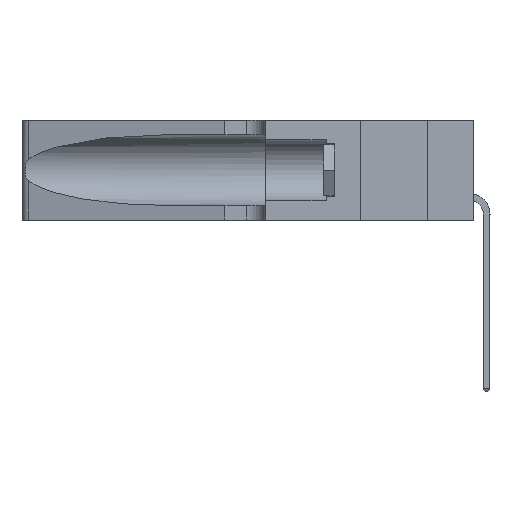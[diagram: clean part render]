
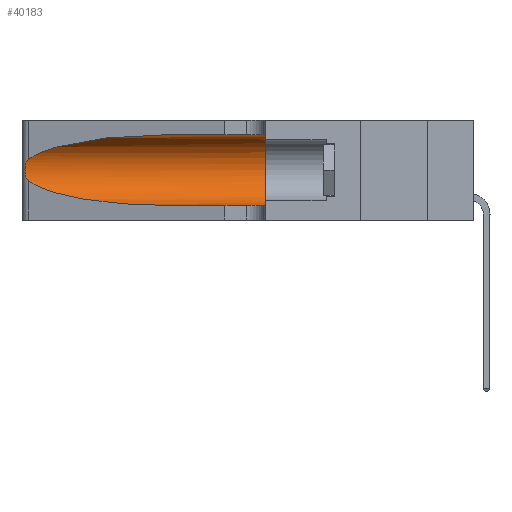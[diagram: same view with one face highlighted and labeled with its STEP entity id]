
A CAD part, left-side view. The second image highlights one B-rep face of the part: STEP entity #40183.
In plain terms, the highlighted cylindrical face has radius 3.308 mm (diameter 6.617 mm), a partial arc.
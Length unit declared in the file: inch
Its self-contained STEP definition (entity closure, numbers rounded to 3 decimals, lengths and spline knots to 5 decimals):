
#824 = LINE ( 'NONE', #29548, #28045 ) ;
#973 = CARTESIAN_POINT ( 'NONE',  ( 0.25487, 1.22718, 0.22369 ) ) ;
#1324 = VECTOR ( 'NONE', #36183, 39.37008 ) ;
#3163 = CARTESIAN_POINT ( 'NONE',  ( 0.25854, 1.2359, 0.20912 ) ) ;
#4702 = CARTESIAN_POINT ( 'NONE',  ( 0.1305, 0.35, 0.05475 ) ) ;
#4826 = ORIENTED_EDGE ( 'NONE', *, *, #31050, .T. ) ;
#7229 = CARTESIAN_POINT ( 'NONE',  ( 0.2373, 1.15595, 0.28018 ) ) ;
#8514 = LINE ( 'NONE', #33286, #1324 ) ;
#10471 = VERTEX_POINT ( 'NONE', #37526 ) ;
#10708 = CARTESIAN_POINT ( 'NONE',  ( 0.25487, 1.22718, 0.14631 ) ) ;
#12821 = DIRECTION ( 'NONE',  ( 0., 0., 1. ) ) ;
#12912 = CARTESIAN_POINT ( 'NONE',  ( 0.18966, 0.96281, 0.05475 ) ) ;
#12975 = CARTESIAN_POINT ( 'NONE',  ( 0.25487, 1.22718, 0.14631 ) ) ;
#13049 = CYLINDRICAL_SURFACE ( 'NONE', #17770, 0.13025 ) ;
#13206 = VERTEX_POINT ( 'NONE', #13548 ) ;
#13548 = CARTESIAN_POINT ( 'NONE',  ( 0.1305, 0.72297, 0.05475 ) ) ;
#15784 = ORIENTED_EDGE ( 'NONE', *, *, #37492, .F. ) ;
#16035 = CARTESIAN_POINT ( 'NONE',  ( 0.26075, 1.23896, 0.178 ) ) ;
#16224 = DIRECTION ( 'NONE',  ( 0., 0., -1. ) ) ;
#16693 = DIRECTION ( 'NONE',  ( 0., -1., 0. ) ) ;
#17770 = AXIS2_PLACEMENT_3D ( 'NONE', #26610, #35866, #16224 ) ;
#18976 = CARTESIAN_POINT ( 'NONE',  ( 0.1305, 0.72297, 0.05475 ) ) ;
#19411 = ORIENTED_EDGE ( 'NONE', *, *, #23525, .T. ) ;
#20201 = CARTESIAN_POINT ( 'NONE',  ( 0.18966, 0.96281, 0.31525 ) ) ;
#20498 = VERTEX_POINT ( 'NONE', #35727 ) ;
#20752 = VERTEX_POINT ( 'NONE', #4702 ) ;
#22020 = VERTEX_POINT ( 'NONE', #973 ) ;
#22325 = CARTESIAN_POINT ( 'NONE',  ( 0.25639, 1.23186, 0.15144 ) ) ;
#22878 = CARTESIAN_POINT ( 'NONE',  ( 0.1305, 0.35, 0.185 ) ) ;
#23478 = CARTESIAN_POINT ( 'NONE',  ( 0.1305, 0.72297, 0.31525 ) ) ;
#23525 = EDGE_CURVE ( 'NONE', #13206, #20752, #824, .T. ) ;
#25500 = EDGE_CURVE ( 'NONE', #20498, #22020, #26716, .T. ) ;
#25588 = CARTESIAN_POINT ( 'NONE',  ( 0.26017, 1.23833, 0.17102 ) ) ;
#25956 = CARTESIAN_POINT ( 'NONE',  ( 0.25487, 1.22718, 0.14631 ) ) ;
#26283 = DIRECTION ( 'NONE',  ( 0., 1., 0. ) ) ;
#26521 = ORIENTED_EDGE ( 'NONE', *, *, #36376, .T. ) ;
#26610 = CARTESIAN_POINT ( 'NONE',  ( 0.1305, 1.61858, 0.185 ) ) ;
#26619 = CARTESIAN_POINT ( 'NONE',  ( 0.25487, 1.22718, 0.22369 ) ) ;
#26694 = EDGE_CURVE ( 'NONE', #20498, #10471, #8514, .T. ) ;
#26716 =( BOUNDED_CURVE ( )  B_SPLINE_CURVE ( 3, ( #23478, #20201, #7229, #26619 ),
 .UNSPECIFIED., .F., .T. ) 
 B_SPLINE_CURVE_WITH_KNOTS ( ( 4, 4 ),
 ( 1.5708, 2.84003 ),
 .UNSPECIFIED. ) 
 CURVE ( )  GEOMETRIC_REPRESENTATION_ITEM ( )  RATIONAL_B_SPLINE_CURVE ( ( 1., 0.87, 0.87, 1. ) ) 
 REPRESENTATION_ITEM ( '' )  );
#27386 = FACE_OUTER_BOUND ( 'NONE', #37531, .T. ) ;
#27489 =( BOUNDED_CURVE ( )  B_SPLINE_CURVE ( 3, ( #25956, #42255, #12912, #18976 ),
 .UNSPECIFIED., .F., .T. ) 
 B_SPLINE_CURVE_WITH_KNOTS ( ( 4, 4 ),
 ( 3.44316, 4.71239 ),
 .UNSPECIFIED. ) 
 CURVE ( )  GEOMETRIC_REPRESENTATION_ITEM ( )  RATIONAL_B_SPLINE_CURVE ( ( 1., 0.87, 0.87, 1. ) ) 
 REPRESENTATION_ITEM ( '' )  );
#28045 = VECTOR ( 'NONE', #16693, 39.37008 ) ;
#28880 = CARTESIAN_POINT ( 'NONE',  ( 0.25555, 1.22994, 0.2215 ) ) ;
#29548 = CARTESIAN_POINT ( 'NONE',  ( 0.1305, 1.61858, 0.05475 ) ) ;
#30541 = ORIENTED_EDGE ( 'NONE', *, *, #26694, .F. ) ;
#31050 = EDGE_CURVE ( 'NONE', #22020, #38394, #36469, .T. ) ;
#32314 = ORIENTED_EDGE ( 'NONE', *, *, #25500, .T. ) ;
#32475 = CARTESIAN_POINT ( 'NONE',  ( 0.25789, 1.23486, 0.15765 ) ) ;
#32757 = CARTESIAN_POINT ( 'NONE',  ( 0.26075, 1.23896, 0.19203 ) ) ;
#33286 = CARTESIAN_POINT ( 'NONE',  ( 0.1305, 1.61858, 0.31525 ) ) ;
#34894 = CIRCLE ( 'NONE', #37502, 0.13025 ) ;
#35661 = CARTESIAN_POINT ( 'NONE',  ( 0.25487, 1.22718, 0.22369 ) ) ;
#35727 = CARTESIAN_POINT ( 'NONE',  ( 0.1305, 0.72297, 0.31525 ) ) ;
#35866 = DIRECTION ( 'NONE',  ( 0., -1., 0. ) ) ;
#36183 = DIRECTION ( 'NONE',  ( 0., -1., 0. ) ) ;
#36376 = EDGE_CURVE ( 'NONE', #38394, #13206, #27489, .T. ) ;
#36469 = B_SPLINE_CURVE_WITH_KNOTS ( 'NONE', 3,
 ( #35661, #28880, #39259, #42604, #3163, #38839, #32757, #16035, #25588, #38973, #32475, #22325, #42166, #12975 ),
 .UNSPECIFIED., .F., .F.,
 ( 4, 2, 2, 2, 2, 2, 4 ),
 ( 0., 0.00027, 0.00053, 0.00107, 0.0016, 0.00187, 0.00214 ),
 .UNSPECIFIED. ) ;
#37492 = EDGE_CURVE ( 'NONE', #10471, #20752, #34894, .T. ) ;
#37502 = AXIS2_PLACEMENT_3D ( 'NONE', #22878, #26283, #12821 ) ;
#37526 = CARTESIAN_POINT ( 'NONE',  ( 0.1305, 0.35, 0.31525 ) ) ;
#37531 = EDGE_LOOP ( 'NONE', ( #32314, #4826, #26521, #19411, #15784, #30541 ) ) ;
#38394 = VERTEX_POINT ( 'NONE', #10708 ) ;
#38839 = CARTESIAN_POINT ( 'NONE',  ( 0.26018, 1.23835, 0.19895 ) ) ;
#38973 = CARTESIAN_POINT ( 'NONE',  ( 0.25856, 1.23593, 0.16098 ) ) ;
#39259 = CARTESIAN_POINT ( 'NONE',  ( 0.25639, 1.23184, 0.21858 ) ) ;
#40183 = ADVANCED_FACE ( 'NONE', ( #27386 ), #13049, .F. ) ;
#42166 = CARTESIAN_POINT ( 'NONE',  ( 0.25555, 1.22993, 0.14849 ) ) ;
#42255 = CARTESIAN_POINT ( 'NONE',  ( 0.2373, 1.15595, 0.08982 ) ) ;
#42604 = CARTESIAN_POINT ( 'NONE',  ( 0.25787, 1.23484, 0.2124 ) ) ;
